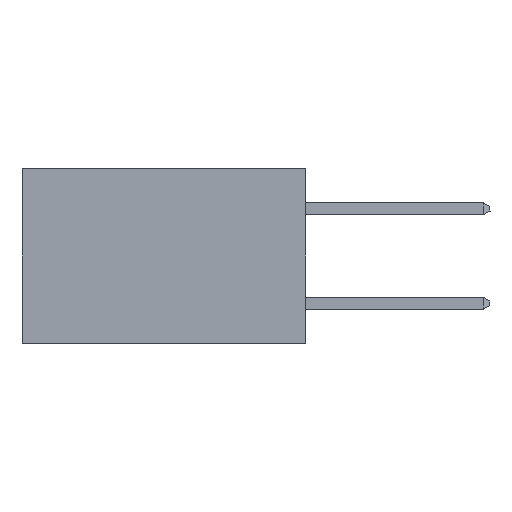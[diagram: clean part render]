
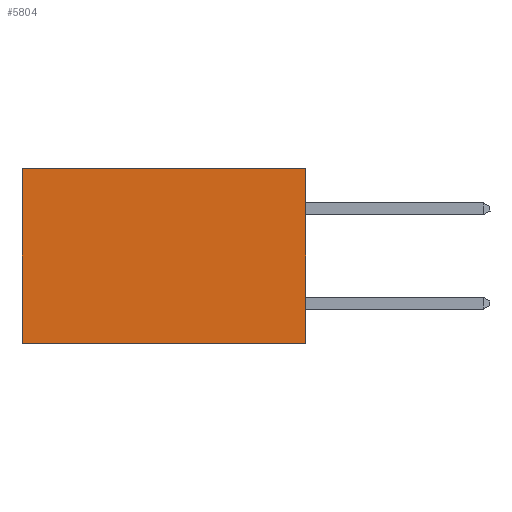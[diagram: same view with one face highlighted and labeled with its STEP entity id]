
A CAD part, left-side view. The second image highlights one B-rep face of the part: STEP entity #5804.
In plain terms, the highlighted planar face has unit normal (-1, 0, 0).
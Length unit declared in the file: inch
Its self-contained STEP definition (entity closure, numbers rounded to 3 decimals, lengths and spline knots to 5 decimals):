
#406 = VECTOR ( 'NONE', #3844, 39.37008 ) ;
#880 = EDGE_CURVE ( 'NONE', #10249, #5841, #3090, .T. ) ;
#2024 = VERTEX_POINT ( 'NONE', #7380 ) ;
#2219 = CARTESIAN_POINT ( 'NONE',  ( 0.298, 0., -0.37 ) ) ;
#2475 = CARTESIAN_POINT ( 'NONE',  ( 0.298, 0., 0. ) ) ;
#2827 = VECTOR ( 'NONE', #9685, 39.37008 ) ;
#2990 = LINE ( 'NONE', #4514, #5369 ) ;
#3090 = LINE ( 'NONE', #12744, #406 ) ;
#3152 = ORIENTED_EDGE ( 'NONE', *, *, #3921, .T. ) ;
#3619 = ORIENTED_EDGE ( 'NONE', *, *, #880, .F. ) ;
#3844 = DIRECTION ( 'NONE',  ( 0., 1., 0. ) ) ;
#3921 = EDGE_CURVE ( 'NONE', #2024, #5841, #2990, .T. ) ;
#3949 = VERTEX_POINT ( 'NONE', #2475 ) ;
#4079 = EDGE_CURVE ( 'NONE', #3949, #10249, #7388, .T. ) ;
#4514 = CARTESIAN_POINT ( 'NONE',  ( 0.298, 0.6, 0. ) ) ;
#4639 = CARTESIAN_POINT ( 'NONE',  ( 0.298, 0., 0. ) ) ;
#4976 = CARTESIAN_POINT ( 'NONE',  ( 0.298, 0., 0. ) ) ;
#5018 = DIRECTION ( 'NONE',  ( 0., 1., 0. ) ) ;
#5080 = DIRECTION ( 'NONE',  ( 1., 0., 0. ) ) ;
#5369 = VECTOR ( 'NONE', #10602, 39.37008 ) ;
#5804 = ADVANCED_FACE ( 'NONE', ( #7033 ), #7137, .F. ) ;
#5841 = VERTEX_POINT ( 'NONE', #9069 ) ;
#6179 = DIRECTION ( 'NONE',  ( 0., 0., -1. ) ) ;
#6782 = EDGE_CURVE ( 'NONE', #3949, #2024, #10561, .T. ) ;
#7033 = FACE_OUTER_BOUND ( 'NONE', #10750, .T. ) ;
#7137 = PLANE ( 'NONE',  #7573 ) ;
#7191 = ORIENTED_EDGE ( 'NONE', *, *, #6782, .T. ) ;
#7380 = CARTESIAN_POINT ( 'NONE',  ( 0.298, 0.6, 0. ) ) ;
#7388 = LINE ( 'NONE', #4639, #2827 ) ;
#7573 = AXIS2_PLACEMENT_3D ( 'NONE', #11020, #5080, #6179 ) ;
#8521 = VECTOR ( 'NONE', #5018, 39.37008 ) ;
#9069 = CARTESIAN_POINT ( 'NONE',  ( 0.298, 0.6, -0.37 ) ) ;
#9685 = DIRECTION ( 'NONE',  ( 0., 0., -1. ) ) ;
#10249 = VERTEX_POINT ( 'NONE', #2219 ) ;
#10561 = LINE ( 'NONE', #4976, #8521 ) ;
#10602 = DIRECTION ( 'NONE',  ( 0., 0., -1. ) ) ;
#10750 = EDGE_LOOP ( 'NONE', ( #3152, #3619, #11319, #7191 ) ) ;
#11020 = CARTESIAN_POINT ( 'NONE',  ( 0.298, 0., 0. ) ) ;
#11319 = ORIENTED_EDGE ( 'NONE', *, *, #4079, .F. ) ;
#12744 = CARTESIAN_POINT ( 'NONE',  ( 0.298, 0., -0.37 ) ) ;
